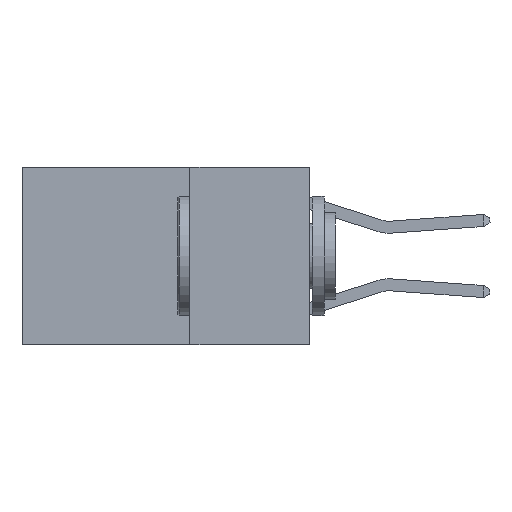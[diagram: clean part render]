
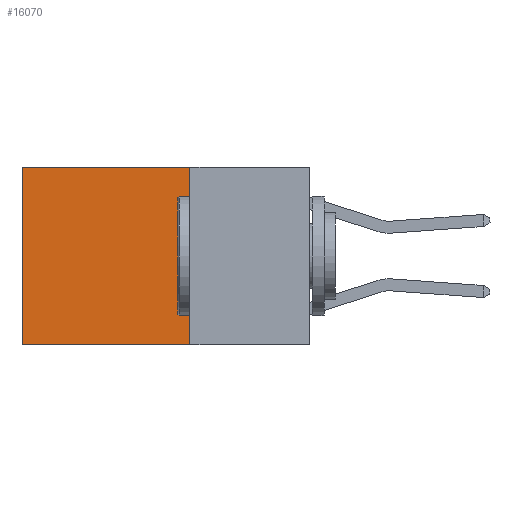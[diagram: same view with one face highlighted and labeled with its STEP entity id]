
A CAD part, left-side view. The second image highlights one B-rep face of the part: STEP entity #16070.
In plain terms, the highlighted planar face has unit normal (-1, 0, 0).
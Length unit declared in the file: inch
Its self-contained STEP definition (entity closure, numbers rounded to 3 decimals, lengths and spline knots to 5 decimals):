
#107 = AXIS2_PLACEMENT_3D ( 'NONE', #727, #12369, #2426 ) ;
#620 = LINE ( 'NONE', #10724, #17259 ) ;
#727 = CARTESIAN_POINT ( 'NONE',  ( 0.2625, 0.25, 0. ) ) ;
#1716 = ORIENTED_EDGE ( 'NONE', *, *, #15828, .T. ) ;
#1756 = CARTESIAN_POINT ( 'NONE',  ( 0.2625, 0.6, 0. ) ) ;
#2426 = DIRECTION ( 'NONE',  ( 0., 0., -1. ) ) ;
#3080 = VERTEX_POINT ( 'NONE', #8976 ) ;
#5346 = ORIENTED_EDGE ( 'NONE', *, *, #14146, .F. ) ;
#5379 = FACE_OUTER_BOUND ( 'NONE', #11373, .T. ) ;
#5699 = CARTESIAN_POINT ( 'NONE',  ( 0.2625, 0.25, 0. ) ) ;
#6975 = CARTESIAN_POINT ( 'NONE',  ( 0.2625, 0.6, 0. ) ) ;
#7408 = PLANE ( 'NONE',  #107 ) ;
#7459 = DIRECTION ( 'NONE',  ( 0., 1., 0. ) ) ;
#8496 = CARTESIAN_POINT ( 'NONE',  ( 0.2625, 0.6, -0.37 ) ) ;
#8976 = CARTESIAN_POINT ( 'NONE',  ( 0.2625, 0.25, 0. ) ) ;
#9326 = CARTESIAN_POINT ( 'NONE',  ( 0.2625, 0.25, -0.37 ) ) ;
#10541 = LINE ( 'NONE', #1756, #14461 ) ;
#10724 = CARTESIAN_POINT ( 'NONE',  ( 0.2625, 0.25, 0. ) ) ;
#11191 = VERTEX_POINT ( 'NONE', #8496 ) ;
#11373 = EDGE_LOOP ( 'NONE', ( #1716, #5346, #16674, #20193 ) ) ;
#12363 = CARTESIAN_POINT ( 'NONE',  ( 0.2625, 0.25, -0.37 ) ) ;
#12369 = DIRECTION ( 'NONE',  ( 1., 0., 0. ) ) ;
#12415 = DIRECTION ( 'NONE',  ( 0., 0., -1. ) ) ;
#12691 = EDGE_CURVE ( 'NONE', #3080, #15904, #17471, .T. ) ;
#14146 = EDGE_CURVE ( 'NONE', #21286, #11191, #19998, .T. ) ;
#14461 = VECTOR ( 'NONE', #15084, 39.37008 ) ;
#15084 = DIRECTION ( 'NONE',  ( 0., 0., -1. ) ) ;
#15657 = VECTOR ( 'NONE', #7459, 39.37008 ) ;
#15828 = EDGE_CURVE ( 'NONE', #15904, #11191, #10541, .T. ) ;
#15904 = VERTEX_POINT ( 'NONE', #6975 ) ;
#16070 = ADVANCED_FACE ( 'NONE', ( #5379 ), #7408, .F. ) ;
#16674 = ORIENTED_EDGE ( 'NONE', *, *, #16796, .F. ) ;
#16796 = EDGE_CURVE ( 'NONE', #3080, #21286, #620, .T. ) ;
#16957 = VECTOR ( 'NONE', #18908, 39.37008 ) ;
#17259 = VECTOR ( 'NONE', #12415, 39.37008 ) ;
#17471 = LINE ( 'NONE', #5699, #16957 ) ;
#18908 = DIRECTION ( 'NONE',  ( 0., 1., 0. ) ) ;
#19998 = LINE ( 'NONE', #12363, #15657 ) ;
#20193 = ORIENTED_EDGE ( 'NONE', *, *, #12691, .T. ) ;
#21286 = VERTEX_POINT ( 'NONE', #9326 ) ;
